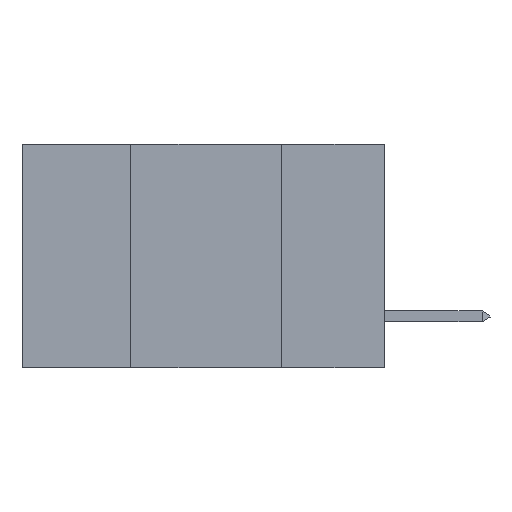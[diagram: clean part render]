
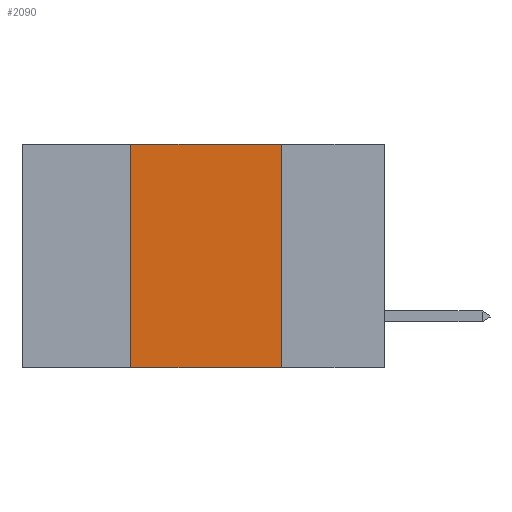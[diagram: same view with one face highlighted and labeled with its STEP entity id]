
A CAD part, left-side view. The second image highlights one B-rep face of the part: STEP entity #2090.
In plain terms, the highlighted planar face has unit normal (-1, 0, 0).
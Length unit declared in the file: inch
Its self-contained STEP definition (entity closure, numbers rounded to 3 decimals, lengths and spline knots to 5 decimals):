
#84 = DIRECTION ( 'NONE',  ( 0., 0., -1. ) ) ;
#116 = VECTOR ( 'NONE', #8767, 39.37008 ) ;
#191 = EDGE_CURVE ( 'NONE', #7999, #4328, #1174, .T. ) ;
#650 = AXIS2_PLACEMENT_3D ( 'NONE', #3559, #4303, #84 ) ;
#756 = DIRECTION ( 'NONE',  ( 0., 0., -1. ) ) ;
#762 = DIRECTION ( 'NONE',  ( 0., -1., 0. ) ) ;
#1174 = LINE ( 'NONE', #2017, #116 ) ;
#2017 = CARTESIAN_POINT ( 'NONE',  ( 0., 0.6, 0. ) ) ;
#2085 = LINE ( 'NONE', #6503, #5527 ) ;
#2090 = ADVANCED_FACE ( 'NONE', ( #5909 ), #3415, .F. ) ;
#2502 = CARTESIAN_POINT ( 'NONE',  ( 0., 0.17, 0. ) ) ;
#2855 = CARTESIAN_POINT ( 'NONE',  ( 0., 0.17, -0.37 ) ) ;
#3045 = VERTEX_POINT ( 'NONE', #2855 ) ;
#3415 = PLANE ( 'NONE',  #650 ) ;
#3530 = CARTESIAN_POINT ( 'NONE',  ( 0., 0.42, 0. ) ) ;
#3559 = CARTESIAN_POINT ( 'NONE',  ( 0., 0.6, 0. ) ) ;
#4303 = DIRECTION ( 'NONE',  ( 1., 0., 0. ) ) ;
#4328 = VERTEX_POINT ( 'NONE', #2502 ) ;
#4713 = ORIENTED_EDGE ( 'NONE', *, *, #191, .F. ) ;
#5157 = ORIENTED_EDGE ( 'NONE', *, *, #5438, .F. ) ;
#5371 = EDGE_LOOP ( 'NONE', ( #5904, #4713, #5157, #10099 ) ) ;
#5438 = EDGE_CURVE ( 'NONE', #6445, #7999, #10418, .T. ) ;
#5527 = VECTOR ( 'NONE', #756, 39.37008 ) ;
#5904 = ORIENTED_EDGE ( 'NONE', *, *, #8890, .F. ) ;
#5909 = FACE_OUTER_BOUND ( 'NONE', #5371, .T. ) ;
#6157 = VECTOR ( 'NONE', #762, 39.37008 ) ;
#6445 = VERTEX_POINT ( 'NONE', #8064 ) ;
#6503 = CARTESIAN_POINT ( 'NONE',  ( 0., 0.17, 0. ) ) ;
#6689 = CARTESIAN_POINT ( 'NONE',  ( 0., 0.42, 0. ) ) ;
#7999 = VERTEX_POINT ( 'NONE', #3530 ) ;
#8064 = CARTESIAN_POINT ( 'NONE',  ( 0., 0.42, -0.37 ) ) ;
#8193 = VECTOR ( 'NONE', #8382, 39.37008 ) ;
#8382 = DIRECTION ( 'NONE',  ( 0., 0., 1. ) ) ;
#8598 = EDGE_CURVE ( 'NONE', #6445, #3045, #9306, .T. ) ;
#8767 = DIRECTION ( 'NONE',  ( 0., -1., 0. ) ) ;
#8890 = EDGE_CURVE ( 'NONE', #4328, #3045, #2085, .T. ) ;
#9258 = CARTESIAN_POINT ( 'NONE',  ( 0., 0.6, -0.37 ) ) ;
#9306 = LINE ( 'NONE', #9258, #6157 ) ;
#10099 = ORIENTED_EDGE ( 'NONE', *, *, #8598, .T. ) ;
#10418 = LINE ( 'NONE', #6689, #8193 ) ;
